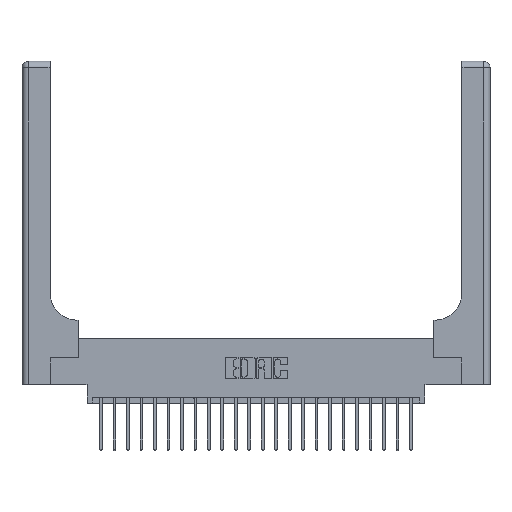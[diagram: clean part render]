
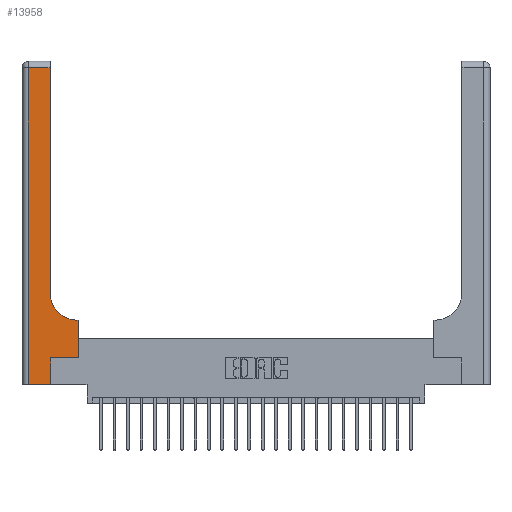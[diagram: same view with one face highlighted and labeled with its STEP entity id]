
A CAD part, top view. The second image highlights one B-rep face of the part: STEP entity #13958.
In plain terms, the highlighted planar face has unit normal (0, 0, 1).
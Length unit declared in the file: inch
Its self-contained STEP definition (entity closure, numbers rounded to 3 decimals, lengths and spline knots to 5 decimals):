
#114 = EDGE_CURVE ( 'NONE', #14278, #9553, #18776, .T. ) ;
#175 = VECTOR ( 'NONE', #22823, 39.37008 ) ;
#652 = CARTESIAN_POINT ( 'NONE',  ( 0.26, 0.6, 0.37 ) ) ;
#938 = AXIS2_PLACEMENT_3D ( 'NONE', #9479, #22186, #11325 ) ;
#1394 = VECTOR ( 'NONE', #5692, 39.37008 ) ;
#1491 = DIRECTION ( 'NONE',  ( 1., 0., 0. ) ) ;
#1622 = EDGE_CURVE ( 'NONE', #12585, #14278, #2509, .T. ) ;
#1660 = CIRCLE ( 'NONE', #938, 0.25 ) ;
#2008 = DIRECTION ( 'NONE',  ( 0., 0., -1. ) ) ;
#2509 = LINE ( 'NONE', #19031, #6738 ) ;
#2739 = CARTESIAN_POINT ( 'NONE',  ( 0.265, 0.25, 0.37 ) ) ;
#3132 = VECTOR ( 'NONE', #16964, 39.37008 ) ;
#3137 = DIRECTION ( 'NONE',  ( 0., 1., 0. ) ) ;
#3748 = LINE ( 'NONE', #652, #7999 ) ;
#3889 = CARTESIAN_POINT ( 'NONE',  ( 0., 0., 0.37 ) ) ;
#4772 = ORIENTED_EDGE ( 'NONE', *, *, #114, .T. ) ;
#5105 = FACE_OUTER_BOUND ( 'NONE', #22376, .T. ) ;
#5127 = VERTEX_POINT ( 'NONE', #6700 ) ;
#5348 = ORIENTED_EDGE ( 'NONE', *, *, #8324, .T. ) ;
#5692 = DIRECTION ( 'NONE',  ( 1., 0., 0. ) ) ;
#5762 = DIRECTION ( 'NONE',  ( -1., 0., 0. ) ) ;
#5838 = LINE ( 'NONE', #19430, #19764 ) ;
#6700 = CARTESIAN_POINT ( 'NONE',  ( 0.528, 0.25, 0.37 ) ) ;
#6738 = VECTOR ( 'NONE', #19190, 39.37008 ) ;
#7799 = VERTEX_POINT ( 'NONE', #16039 ) ;
#7999 = VECTOR ( 'NONE', #22281, 39.37008 ) ;
#8324 = EDGE_CURVE ( 'NONE', #20682, #5127, #22422, .T. ) ;
#8434 = ORIENTED_EDGE ( 'NONE', *, *, #22946, .T. ) ;
#8503 = VECTOR ( 'NONE', #5762, 39.37008 ) ;
#8658 = CARTESIAN_POINT ( 'NONE',  ( 0.265, 0.25, 0.37 ) ) ;
#9479 = CARTESIAN_POINT ( 'NONE',  ( 0.51, 0.85, 0.37 ) ) ;
#9499 = VERTEX_POINT ( 'NONE', #21209 ) ;
#9553 = VERTEX_POINT ( 'NONE', #21503 ) ;
#9792 = LINE ( 'NONE', #11969, #175 ) ;
#10654 = EDGE_CURVE ( 'NONE', #7799, #20682, #5838, .T. ) ;
#10655 = ORIENTED_EDGE ( 'NONE', *, *, #18211, .T. ) ;
#11325 = DIRECTION ( 'NONE',  ( 1., 0., 0. ) ) ;
#11466 = CARTESIAN_POINT ( 'NONE',  ( 0.06, 3., 0.37 ) ) ;
#11790 = CARTESIAN_POINT ( 'NONE',  ( 0., 2.94, 0.37 ) ) ;
#11969 = CARTESIAN_POINT ( 'NONE',  ( 0.528, 0.25, 0.37 ) ) ;
#12277 = CARTESIAN_POINT ( 'NONE',  ( 0.26, 0.85, 0.37 ) ) ;
#12372 = PLANE ( 'NONE',  #16252 ) ;
#12585 = VERTEX_POINT ( 'NONE', #12277 ) ;
#13688 = CARTESIAN_POINT ( 'NONE',  ( 0.51, 0.6, 0.37 ) ) ;
#13958 = ADVANCED_FACE ( 'NONE', ( #5105 ), #12372, .F. ) ;
#14278 = VERTEX_POINT ( 'NONE', #19074 ) ;
#14708 = DIRECTION ( 'NONE',  ( -1., 0., 0. ) ) ;
#15144 = EDGE_CURVE ( 'NONE', #9553, #9499, #22436, .T. ) ;
#15879 = LINE ( 'NONE', #3889, #1394 ) ;
#16039 = CARTESIAN_POINT ( 'NONE',  ( 0.265, 0., 0.37 ) ) ;
#16252 = AXIS2_PLACEMENT_3D ( 'NONE', #20099, #2008, #14708 ) ;
#16277 = VERTEX_POINT ( 'NONE', #18336 ) ;
#16364 = EDGE_CURVE ( 'NONE', #18583, #12585, #1660, .T. ) ;
#16964 = DIRECTION ( 'NONE',  ( 0., -1., 0. ) ) ;
#17641 = VECTOR ( 'NONE', #1491, 39.37008 ) ;
#18211 = EDGE_CURVE ( 'NONE', #5127, #16277, #9792, .T. ) ;
#18336 = CARTESIAN_POINT ( 'NONE',  ( 0.528, 0.6, 0.37 ) ) ;
#18583 = VERTEX_POINT ( 'NONE', #13688 ) ;
#18776 = LINE ( 'NONE', #11790, #8503 ) ;
#19031 = CARTESIAN_POINT ( 'NONE',  ( 0.26, 3., 0.37 ) ) ;
#19074 = CARTESIAN_POINT ( 'NONE',  ( 0.26, 2.94, 0.37 ) ) ;
#19190 = DIRECTION ( 'NONE',  ( 0., 1., 0. ) ) ;
#19257 = ORIENTED_EDGE ( 'NONE', *, *, #1622, .T. ) ;
#19430 = CARTESIAN_POINT ( 'NONE',  ( 0.265, 0., 0.37 ) ) ;
#19749 = EDGE_CURVE ( 'NONE', #16277, #18583, #3748, .T. ) ;
#19764 = VECTOR ( 'NONE', #3137, 39.37008 ) ;
#20099 = CARTESIAN_POINT ( 'NONE',  ( 0., 3., 0.37 ) ) ;
#20682 = VERTEX_POINT ( 'NONE', #2739 ) ;
#21209 = CARTESIAN_POINT ( 'NONE',  ( 0.06, 0., 0.37 ) ) ;
#21430 = ORIENTED_EDGE ( 'NONE', *, *, #15144, .T. ) ;
#21503 = CARTESIAN_POINT ( 'NONE',  ( 0.06, 2.94, 0.37 ) ) ;
#21843 = ORIENTED_EDGE ( 'NONE', *, *, #16364, .T. ) ;
#22084 = ORIENTED_EDGE ( 'NONE', *, *, #10654, .T. ) ;
#22186 = DIRECTION ( 'NONE',  ( 0., 0., -1. ) ) ;
#22262 = ORIENTED_EDGE ( 'NONE', *, *, #19749, .T. ) ;
#22281 = DIRECTION ( 'NONE',  ( -1., 0., 0. ) ) ;
#22376 = EDGE_LOOP ( 'NONE', ( #19257, #4772, #21430, #8434, #22084, #5348, #10655, #22262, #21843 ) ) ;
#22422 = LINE ( 'NONE', #8658, #17641 ) ;
#22436 = LINE ( 'NONE', #11466, #3132 ) ;
#22823 = DIRECTION ( 'NONE',  ( 0., 1., 0. ) ) ;
#22946 = EDGE_CURVE ( 'NONE', #9499, #7799, #15879, .T. ) ;
